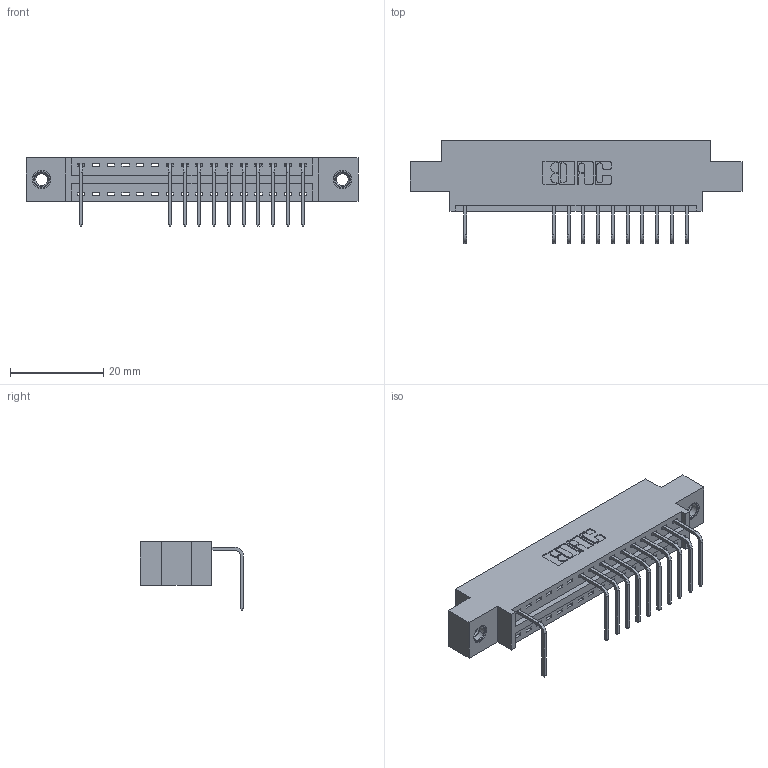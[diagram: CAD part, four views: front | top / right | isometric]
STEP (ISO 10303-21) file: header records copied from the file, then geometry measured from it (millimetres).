
FILE_DESCRIPTION (( 'STEP AP203' ), '1' );
FILE_NAME ('346-016-558-607.STEP', '2018-08-20T05:10:37', ( '' ), ( '' ), 'SwSTEP 2.0', 'SolidWorks 2016', '' );
FILE_SCHEMA (( 'CONFIG_CONTROL_DESIGN' ));
Length unit declared in the file: inch
Products named in the file (4): 346 Part_0.170 Offset - 0.156 Dia-TI; 345-292-001_558 Tail - 2; 345-250-001_345-250-005-103; 346-016-558-607
Assembly tree (14 placements, depth 2):
  346-016-558-607
    346 Part_0.170 Offset - 0.156 Dia-TI
    345-292-001_558 Tail - 2  x11
    345-250-001_345-250-005-103  x2
Bounding box: 71.37 x 22.16 x 14.73 mm (x, y, z)
Volume: 6464.3 mm3; surface area: 7904.9 mm2
Topology: 14 solids, 14 shells, 906 faces, 2689 edges, 1770 vertices
Faces by surface type: plane 624, cylinder 266, cone 12, torus 4
Entity records: 14672 total; most frequent: CARTESIAN_POINT 2530, ORIENTED_EDGE 2478, DIRECTION 2283, EDGE_CURVE 1239, VECTOR 1023, LINE 1023, VERTEX_POINT 820, AXIS2_PLACEMENT_3D 630
